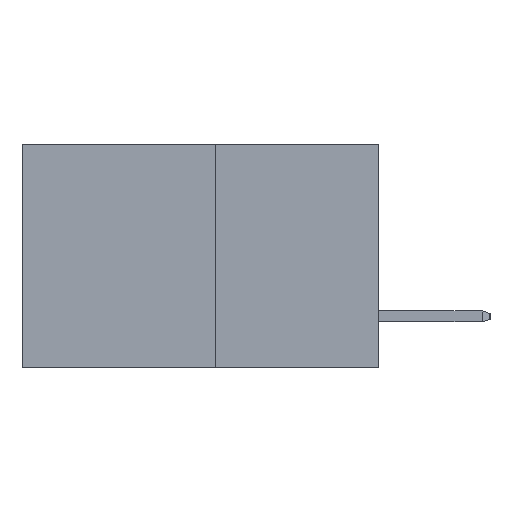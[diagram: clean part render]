
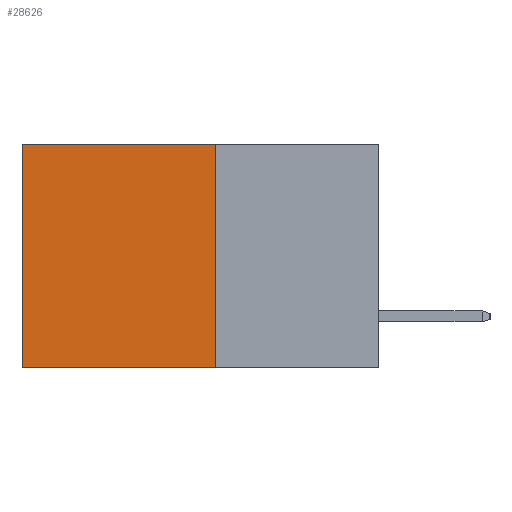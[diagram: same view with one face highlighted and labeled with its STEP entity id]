
A CAD part, left-side view. The second image highlights one B-rep face of the part: STEP entity #28626.
In plain terms, the highlighted planar face has unit normal (-1, 0, 0).
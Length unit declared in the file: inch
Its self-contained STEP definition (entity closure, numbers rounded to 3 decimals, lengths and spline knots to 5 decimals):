
#100 = LINE ( 'NONE', #23919, #10212 ) ;
#262 = DIRECTION ( 'NONE',  ( 0., 1., 0. ) ) ;
#2453 = FACE_OUTER_BOUND ( 'NONE', #4693, .T. ) ;
#2599 = VECTOR ( 'NONE', #14203, 39.37008 ) ;
#2919 = LINE ( 'NONE', #16356, #8345 ) ;
#3907 = CARTESIAN_POINT ( 'NONE',  ( 0.277, 0.27, -0.37 ) ) ;
#4693 = EDGE_LOOP ( 'NONE', ( #6858, #21193, #15264, #19181 ) ) ;
#5843 = AXIS2_PLACEMENT_3D ( 'NONE', #3907, #19956, #6255 ) ;
#6255 = DIRECTION ( 'NONE',  ( 0., 0., -1. ) ) ;
#6858 = ORIENTED_EDGE ( 'NONE', *, *, #21940, .T. ) ;
#7274 = CARTESIAN_POINT ( 'NONE',  ( 0.277, 0.59, -0.37 ) ) ;
#7438 = VERTEX_POINT ( 'NONE', #10123 ) ;
#8272 = VERTEX_POINT ( 'NONE', #24158 ) ;
#8345 = VECTOR ( 'NONE', #262, 39.37008 ) ;
#8750 = LINE ( 'NONE', #7274, #2599 ) ;
#8995 = EDGE_CURVE ( 'NONE', #8272, #21722, #16652, .T. ) ;
#10123 = CARTESIAN_POINT ( 'NONE',  ( 0.277, 0.27, 0. ) ) ;
#10212 = VECTOR ( 'NONE', #24006, 39.37008 ) ;
#12498 = EDGE_CURVE ( 'NONE', #7438, #8272, #100, .T. ) ;
#14203 = DIRECTION ( 'NONE',  ( 0., 0., -1. ) ) ;
#15264 = ORIENTED_EDGE ( 'NONE', *, *, #12498, .F. ) ;
#15330 = CARTESIAN_POINT ( 'NONE',  ( 0.277, 0.27, -0.37 ) ) ;
#15377 = PLANE ( 'NONE',  #5843 ) ;
#16356 = CARTESIAN_POINT ( 'NONE',  ( 0.277, 0.27, 0. ) ) ;
#16652 = LINE ( 'NONE', #15330, #27195 ) ;
#19181 = ORIENTED_EDGE ( 'NONE', *, *, #22585, .T. ) ;
#19956 = DIRECTION ( 'NONE',  ( 1., 0., 0. ) ) ;
#21185 = VERTEX_POINT ( 'NONE', #26753 ) ;
#21193 = ORIENTED_EDGE ( 'NONE', *, *, #8995, .F. ) ;
#21722 = VERTEX_POINT ( 'NONE', #27028 ) ;
#21940 = EDGE_CURVE ( 'NONE', #21185, #21722, #8750, .T. ) ;
#22585 = EDGE_CURVE ( 'NONE', #7438, #21185, #2919, .T. ) ;
#23919 = CARTESIAN_POINT ( 'NONE',  ( 0.277, 0.27, -0.37 ) ) ;
#24006 = DIRECTION ( 'NONE',  ( 0., 0., -1. ) ) ;
#24158 = CARTESIAN_POINT ( 'NONE',  ( 0.277, 0.27, -0.37 ) ) ;
#26753 = CARTESIAN_POINT ( 'NONE',  ( 0.277, 0.59, 0. ) ) ;
#27028 = CARTESIAN_POINT ( 'NONE',  ( 0.277, 0.59, -0.37 ) ) ;
#27195 = VECTOR ( 'NONE', #28808, 39.37008 ) ;
#28626 = ADVANCED_FACE ( 'NONE', ( #2453 ), #15377, .F. ) ;
#28808 = DIRECTION ( 'NONE',  ( 0., 1., 0. ) ) ;
